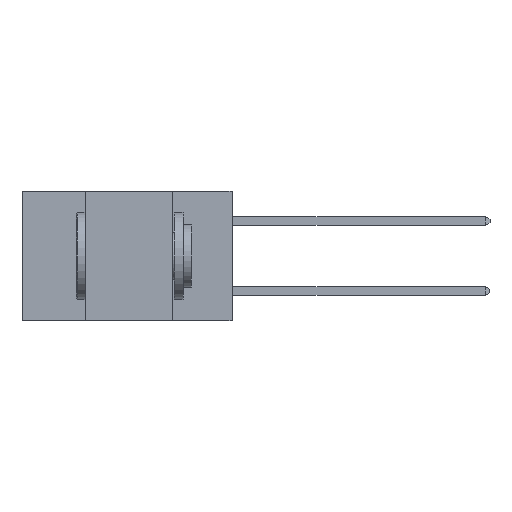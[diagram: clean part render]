
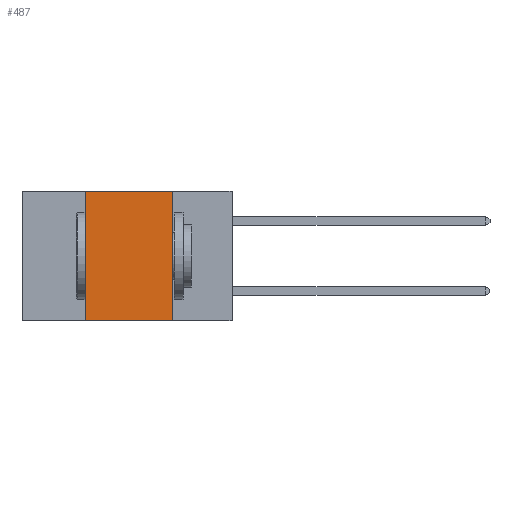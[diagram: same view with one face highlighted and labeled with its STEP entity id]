
A CAD part, left-side view. The second image highlights one B-rep face of the part: STEP entity #487.
In plain terms, the highlighted planar face has unit normal (-1, 0, 0).
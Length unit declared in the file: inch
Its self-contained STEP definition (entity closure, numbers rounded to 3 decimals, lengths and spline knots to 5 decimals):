
#487 = ADVANCED_FACE ( 'NONE', ( #7457 ), #8315, .F. ) ;
#663 = ORIENTED_EDGE ( 'NONE', *, *, #4948, .F. ) ;
#871 = LINE ( 'NONE', #14230, #16915 ) ;
#1149 = ORIENTED_EDGE ( 'NONE', *, *, #4437, .F. ) ;
#1203 = VERTEX_POINT ( 'NONE', #15887 ) ;
#1309 = EDGE_CURVE ( 'NONE', #8061, #9062, #4844, .T. ) ;
#2438 = EDGE_CURVE ( 'NONE', #8061, #5891, #13208, .T. ) ;
#2469 = DIRECTION ( 'NONE',  ( 0., -1., 0. ) ) ;
#2509 = CARTESIAN_POINT ( 'NONE',  ( 0., 0.6, -0.37 ) ) ;
#4437 = EDGE_CURVE ( 'NONE', #9062, #1203, #14814, .T. ) ;
#4543 = CARTESIAN_POINT ( 'NONE',  ( 0., 0.6, 0. ) ) ;
#4633 = DIRECTION ( 'NONE',  ( 0., -1., 0. ) ) ;
#4844 = LINE ( 'NONE', #9923, #16898 ) ;
#4948 = EDGE_CURVE ( 'NONE', #1203, #5891, #871, .T. ) ;
#5193 = DIRECTION ( 'NONE',  ( 0., 0., -1. ) ) ;
#5208 = VECTOR ( 'NONE', #2469, 39.37008 ) ;
#5891 = VERTEX_POINT ( 'NONE', #19060 ) ;
#7457 = FACE_OUTER_BOUND ( 'NONE', #16691, .T. ) ;
#8061 = VERTEX_POINT ( 'NONE', #14440 ) ;
#8138 = DIRECTION ( 'NONE',  ( 0., 0., -1. ) ) ;
#8174 = DIRECTION ( 'NONE',  ( 1., 0., 0. ) ) ;
#8315 = PLANE ( 'NONE',  #19134 ) ;
#8692 = CARTESIAN_POINT ( 'NONE',  ( 0., 0.6, 0. ) ) ;
#9062 = VERTEX_POINT ( 'NONE', #10963 ) ;
#9923 = CARTESIAN_POINT ( 'NONE',  ( 0., 0.42, 0. ) ) ;
#9951 = DIRECTION ( 'NONE',  ( 0., 0., 1. ) ) ;
#10014 = ORIENTED_EDGE ( 'NONE', *, *, #1309, .F. ) ;
#10963 = CARTESIAN_POINT ( 'NONE',  ( 0., 0.42, 0. ) ) ;
#11429 = ORIENTED_EDGE ( 'NONE', *, *, #2438, .T. ) ;
#13208 = LINE ( 'NONE', #2509, #5208 ) ;
#14230 = CARTESIAN_POINT ( 'NONE',  ( 0., 0.17, 0. ) ) ;
#14336 = VECTOR ( 'NONE', #4633, 39.37008 ) ;
#14440 = CARTESIAN_POINT ( 'NONE',  ( 0., 0.42, -0.37 ) ) ;
#14814 = LINE ( 'NONE', #4543, #14336 ) ;
#15887 = CARTESIAN_POINT ( 'NONE',  ( 0., 0.17, 0. ) ) ;
#16691 = EDGE_LOOP ( 'NONE', ( #663, #1149, #10014, #11429 ) ) ;
#16898 = VECTOR ( 'NONE', #9951, 39.37008 ) ;
#16915 = VECTOR ( 'NONE', #5193, 39.37008 ) ;
#19060 = CARTESIAN_POINT ( 'NONE',  ( 0., 0.17, -0.37 ) ) ;
#19134 = AXIS2_PLACEMENT_3D ( 'NONE', #8692, #8174, #8138 ) ;
